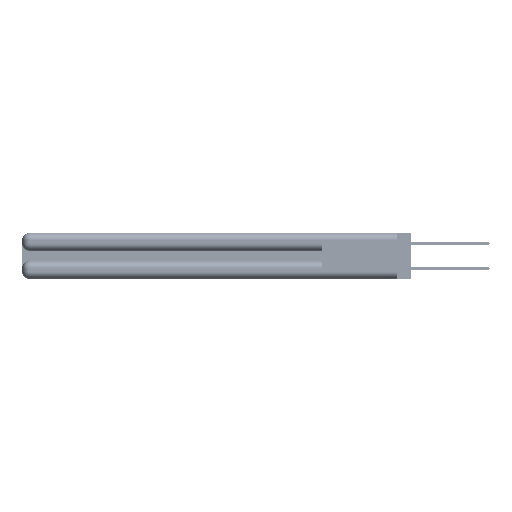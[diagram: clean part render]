
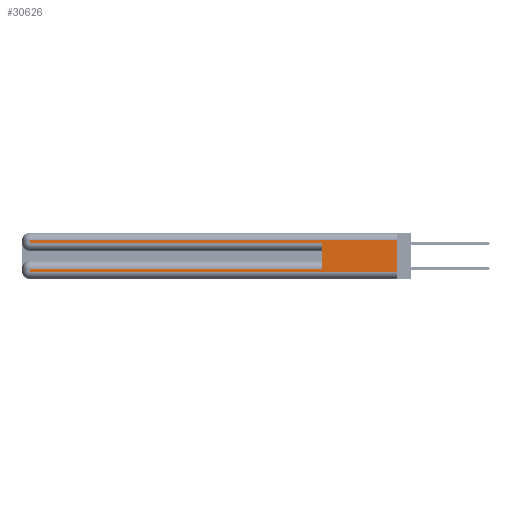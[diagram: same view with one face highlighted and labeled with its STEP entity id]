
A CAD part, left-side view. The second image highlights one B-rep face of the part: STEP entity #30626.
In plain terms, the highlighted planar face has unit normal (-1, 0, 0).
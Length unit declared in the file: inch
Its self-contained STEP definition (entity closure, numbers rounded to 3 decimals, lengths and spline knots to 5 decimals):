
#478 = EDGE_CURVE ( 'NONE', #43275, #24137, #1633, .T. ) ;
#728 = CARTESIAN_POINT ( 'NONE',  ( 0., 0., 0.37 ) ) ;
#1297 = DIRECTION ( 'NONE',  ( 0., 0., -1. ) ) ;
#1486 = CARTESIAN_POINT ( 'NONE',  ( 0., 2.94, 0.06 ) ) ;
#1633 = LINE ( 'NONE', #47851, #34820 ) ;
#1668 = CARTESIAN_POINT ( 'NONE',  ( 0., 2.94, 0.37 ) ) ;
#2998 = CARTESIAN_POINT ( 'NONE',  ( 0., 2.94, 0.37 ) ) ;
#4436 = CARTESIAN_POINT ( 'NONE',  ( 0., 0.6, 0.285 ) ) ;
#4704 = VERTEX_POINT ( 'NONE', #7264 ) ;
#5578 = EDGE_CURVE ( 'NONE', #4704, #29331, #44323, .T. ) ;
#5847 = ORIENTED_EDGE ( 'NONE', *, *, #29075, .T. ) ;
#6687 = ORIENTED_EDGE ( 'NONE', *, *, #25254, .F. ) ;
#6985 = DIRECTION ( 'NONE',  ( 0., 0., 1. ) ) ;
#7084 = VERTEX_POINT ( 'NONE', #1486 ) ;
#7264 = CARTESIAN_POINT ( 'NONE',  ( 0., 0., 0.31 ) ) ;
#8298 = LINE ( 'NONE', #2998, #40039 ) ;
#9939 = VECTOR ( 'NONE', #31018, 39.37008 ) ;
#10003 = ORIENTED_EDGE ( 'NONE', *, *, #478, .T. ) ;
#11873 = CARTESIAN_POINT ( 'NONE',  ( 0., 0., 0.06 ) ) ;
#13961 = CARTESIAN_POINT ( 'NONE',  ( 0., 2.94, 0.285 ) ) ;
#14047 = EDGE_CURVE ( 'NONE', #7084, #29331, #16415, .T. ) ;
#15328 = LINE ( 'NONE', #41523, #48355 ) ;
#15965 = CARTESIAN_POINT ( 'NONE',  ( 0., 0., 0.37 ) ) ;
#16056 = CARTESIAN_POINT ( 'NONE',  ( 0., 0., 0.06 ) ) ;
#16266 = AXIS2_PLACEMENT_3D ( 'NONE', #15965, #46135, #20330 ) ;
#16415 = LINE ( 'NONE', #11873, #26535 ) ;
#17646 = CARTESIAN_POINT ( 'NONE',  ( 0., 2.94, 0.085 ) ) ;
#18305 = EDGE_CURVE ( 'NONE', #4704, #42552, #34733, .T. ) ;
#19366 = ORIENTED_EDGE ( 'NONE', *, *, #18305, .T. ) ;
#20330 = DIRECTION ( 'NONE',  ( 0., 0., -1. ) ) ;
#22087 = DIRECTION ( 'NONE',  ( 0., -1., 0. ) ) ;
#22380 = CARTESIAN_POINT ( 'NONE',  ( 0., 0., 0.085 ) ) ;
#23220 = VECTOR ( 'NONE', #33660, 39.37008 ) ;
#24137 = VERTEX_POINT ( 'NONE', #4436 ) ;
#24724 = DIRECTION ( 'NONE',  ( 0., 0., -1. ) ) ;
#25254 = EDGE_CURVE ( 'NONE', #42156, #24137, #15328, .T. ) ;
#25997 = VECTOR ( 'NONE', #52630, 39.37008 ) ;
#26417 = EDGE_CURVE ( 'NONE', #42156, #34816, #48884, .T. ) ;
#26535 = VECTOR ( 'NONE', #54942, 39.37008 ) ;
#28037 = ORIENTED_EDGE ( 'NONE', *, *, #5578, .F. ) ;
#28809 = PLANE ( 'NONE',  #16266 ) ;
#28928 = CARTESIAN_POINT ( 'NONE',  ( 0., 0., 0.31 ) ) ;
#29075 = EDGE_CURVE ( 'NONE', #34816, #7084, #44661, .T. ) ;
#29331 = VERTEX_POINT ( 'NONE', #16056 ) ;
#30054 = CARTESIAN_POINT ( 'NONE',  ( 0., 2.94, 0.31 ) ) ;
#30626 = ADVANCED_FACE ( 'NONE', ( #43243 ), #28809, .F. ) ;
#31018 = DIRECTION ( 'NONE',  ( 0., 0., -1. ) ) ;
#31880 = VECTOR ( 'NONE', #1297, 39.37008 ) ;
#31976 = CARTESIAN_POINT ( 'NONE',  ( 0., 0.6, 0.085 ) ) ;
#33660 = DIRECTION ( 'NONE',  ( 0., 1., 0. ) ) ;
#34733 = LINE ( 'NONE', #28928, #23220 ) ;
#34762 = ORIENTED_EDGE ( 'NONE', *, *, #35861, .T. ) ;
#34816 = VERTEX_POINT ( 'NONE', #17646 ) ;
#34820 = VECTOR ( 'NONE', #22087, 39.37008 ) ;
#35785 = ORIENTED_EDGE ( 'NONE', *, *, #26417, .T. ) ;
#35861 = EDGE_CURVE ( 'NONE', #42552, #43275, #8298, .T. ) ;
#40039 = VECTOR ( 'NONE', #24724, 39.37008 ) ;
#41523 = CARTESIAN_POINT ( 'NONE',  ( 0., 0.6, 0.145 ) ) ;
#42156 = VERTEX_POINT ( 'NONE', #31976 ) ;
#42552 = VERTEX_POINT ( 'NONE', #30054 ) ;
#43243 = FACE_OUTER_BOUND ( 'NONE', #45212, .T. ) ;
#43275 = VERTEX_POINT ( 'NONE', #13961 ) ;
#44323 = LINE ( 'NONE', #728, #9939 ) ;
#44661 = LINE ( 'NONE', #1668, #31880 ) ;
#44671 = ORIENTED_EDGE ( 'NONE', *, *, #14047, .T. ) ;
#45212 = EDGE_LOOP ( 'NONE', ( #28037, #19366, #34762, #10003, #6687, #35785, #5847, #44671 ) ) ;
#46135 = DIRECTION ( 'NONE',  ( 1., 0., 0. ) ) ;
#47851 = CARTESIAN_POINT ( 'NONE',  ( 0., 0., 0.285 ) ) ;
#48355 = VECTOR ( 'NONE', #6985, 39.37008 ) ;
#48884 = LINE ( 'NONE', #22380, #25997 ) ;
#52630 = DIRECTION ( 'NONE',  ( 0., 1., 0. ) ) ;
#54942 = DIRECTION ( 'NONE',  ( 0., -1., 0. ) ) ;
